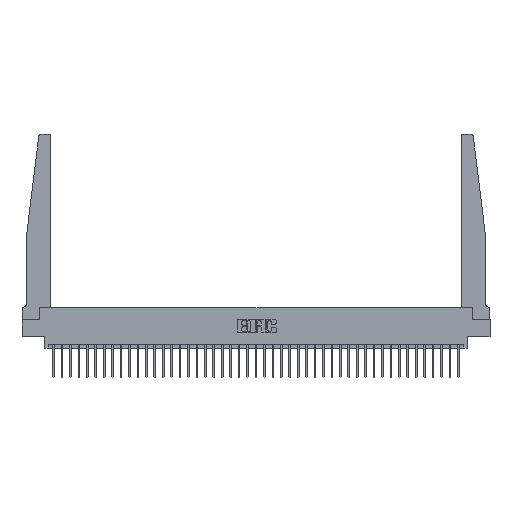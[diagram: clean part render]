
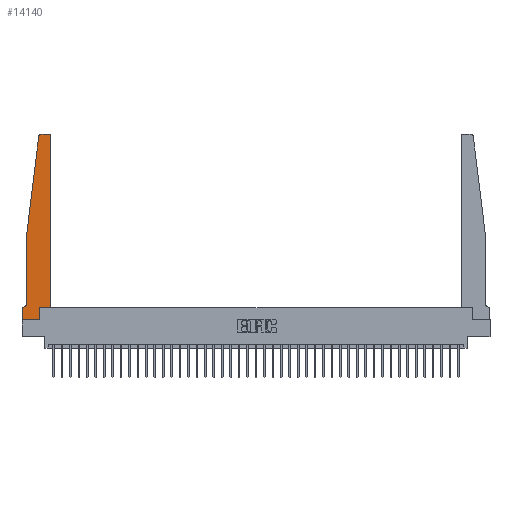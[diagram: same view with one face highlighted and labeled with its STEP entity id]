
A CAD part, top view. The second image highlights one B-rep face of the part: STEP entity #14140.
In plain terms, the highlighted planar face has unit normal (0, 0, 1).
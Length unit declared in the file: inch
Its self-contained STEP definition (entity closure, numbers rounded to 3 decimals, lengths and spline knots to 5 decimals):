
#313 = DIRECTION ( 'NONE',  ( 0., 1., 0. ) ) ;
#480 = EDGE_CURVE ( 'NONE', #21178, #12485, #6880, .T. ) ;
#912 = VERTEX_POINT ( 'NONE', #19153 ) ;
#1433 = DIRECTION ( 'NONE',  ( 0., 0., 1. ) ) ;
#2282 = LINE ( 'NONE', #14441, #31007 ) ;
#2544 = ORIENTED_EDGE ( 'NONE', *, *, #6429, .T. ) ;
#2785 = ORIENTED_EDGE ( 'NONE', *, *, #4045, .T. ) ;
#4045 = EDGE_CURVE ( 'NONE', #18976, #19188, #12335, .T. ) ;
#4588 = ORIENTED_EDGE ( 'NONE', *, *, #19370, .T. ) ;
#4619 = CARTESIAN_POINT ( 'NONE',  ( 0.015, 0.2375, 0.37 ) ) ;
#6387 = LINE ( 'NONE', #34584, #21199 ) ;
#6429 = EDGE_CURVE ( 'NONE', #912, #9850, #34112, .T. ) ;
#6644 = ORIENTED_EDGE ( 'NONE', *, *, #29822, .T. ) ;
#6880 = LINE ( 'NONE', #25906, #16068 ) ;
#7078 = CARTESIAN_POINT ( 'NONE',  ( 0., 0.1875, 0.37 ) ) ;
#7339 = EDGE_CURVE ( 'NONE', #9850, #21178, #26303, .T. ) ;
#7486 = DIRECTION ( 'NONE',  ( -1., 0., 0. ) ) ;
#7758 = CARTESIAN_POINT ( 'NONE',  ( 0.065, 0.2375, 0.37 ) ) ;
#7818 = CARTESIAN_POINT ( 'NONE',  ( 0.2605, 0., 0.37 ) ) ;
#8088 = CARTESIAN_POINT ( 'NONE',  ( 0.065, 1.25, 0.37 ) ) ;
#8310 = FACE_OUTER_BOUND ( 'NONE', #12011, .T. ) ;
#8374 = VECTOR ( 'NONE', #34405, 39.37008 ) ;
#8578 = EDGE_CURVE ( 'NONE', #16094, #34304, #25097, .T. ) ;
#8755 = CARTESIAN_POINT ( 'NONE',  ( 0.425, 0.18, 0.37 ) ) ;
#8774 = AXIS2_PLACEMENT_3D ( 'NONE', #15777, #34956, #18520 ) ;
#9122 = CARTESIAN_POINT ( 'NONE',  ( 0.015, 0.1875, 0.37 ) ) ;
#9349 = DIRECTION ( 'NONE',  ( 1., 0., 0. ) ) ;
#9678 = VERTEX_POINT ( 'NONE', #17785 ) ;
#9850 = VERTEX_POINT ( 'NONE', #7818 ) ;
#10048 = ORIENTED_EDGE ( 'NONE', *, *, #32383, .T. ) ;
#10500 = CARTESIAN_POINT ( 'NONE',  ( 0.065, 0.1875, 0.37 ) ) ;
#11007 = VERTEX_POINT ( 'NONE', #26734 ) ;
#11939 = CARTESIAN_POINT ( 'NONE',  ( 0.2605, 0.18, 0.37 ) ) ;
#12011 = EDGE_LOOP ( 'NONE', ( #32523, #6644, #2785, #13291, #15562, #20922, #10048, #2544, #18389, #19428, #4588, #18630 ) ) ;
#12020 = DIRECTION ( 'NONE',  ( 0., 0., 1. ) ) ;
#12335 = LINE ( 'NONE', #18203, #19683 ) ;
#12485 = VERTEX_POINT ( 'NONE', #8755 ) ;
#13291 = ORIENTED_EDGE ( 'NONE', *, *, #17064, .T. ) ;
#14013 = VECTOR ( 'NONE', #21661, 39.37008 ) ;
#14140 = ADVANCED_FACE ( 'NONE', ( #8310 ), #15522, .T. ) ;
#14441 = CARTESIAN_POINT ( 'NONE',  ( 0.425, 0.18, 0.37 ) ) ;
#14800 = VECTOR ( 'NONE', #31903, 39.37008 ) ;
#15348 = CIRCLE ( 'NONE', #25427, 0.03 ) ;
#15453 = CARTESIAN_POINT ( 'NONE',  ( 0.065, 1.25, 0.37 ) ) ;
#15522 = PLANE ( 'NONE',  #33611 ) ;
#15562 = ORIENTED_EDGE ( 'NONE', *, *, #22036, .T. ) ;
#15777 = CARTESIAN_POINT ( 'NONE',  ( 0.395, 2.72, 0.37 ) ) ;
#15808 = LINE ( 'NONE', #31666, #8374 ) ;
#16068 = VECTOR ( 'NONE', #9349, 39.37008 ) ;
#16094 = VERTEX_POINT ( 'NONE', #29824 ) ;
#16121 = EDGE_CURVE ( 'NONE', #16365, #11007, #29520, .T. ) ;
#16365 = VERTEX_POINT ( 'NONE', #9122 ) ;
#16537 = AXIS2_PLACEMENT_3D ( 'NONE', #4619, #24102, #7486 ) ;
#17064 = EDGE_CURVE ( 'NONE', #19188, #31358, #22991, .T. ) ;
#17785 = CARTESIAN_POINT ( 'NONE',  ( 0.27653, 2.75, 0.37 ) ) ;
#18137 = DIRECTION ( 'NONE',  ( 0., -1., 0. ) ) ;
#18203 = CARTESIAN_POINT ( 'NONE',  ( 0.065, 1.25, 0.37 ) ) ;
#18389 = ORIENTED_EDGE ( 'NONE', *, *, #7339, .T. ) ;
#18520 = DIRECTION ( 'NONE',  ( 1., 0., 0. ) ) ;
#18630 = ORIENTED_EDGE ( 'NONE', *, *, #8578, .T. ) ;
#18976 = VERTEX_POINT ( 'NONE', #34748 ) ;
#19153 = CARTESIAN_POINT ( 'NONE',  ( 0., 0., 0.37 ) ) ;
#19188 = VERTEX_POINT ( 'NONE', #8088 ) ;
#19370 = EDGE_CURVE ( 'NONE', #12485, #16094, #2282, .T. ) ;
#19428 = ORIENTED_EDGE ( 'NONE', *, *, #480, .T. ) ;
#19683 = VECTOR ( 'NONE', #34657, 39.37008 ) ;
#19742 = CARTESIAN_POINT ( 'NONE',  ( 0., 0., 0.37 ) ) ;
#19863 = VECTOR ( 'NONE', #24046, 39.37008 ) ;
#20922 = ORIENTED_EDGE ( 'NONE', *, *, #16121, .T. ) ;
#21063 = DIRECTION ( 'NONE',  ( 1., 0., 0. ) ) ;
#21178 = VERTEX_POINT ( 'NONE', #11939 ) ;
#21199 = VECTOR ( 'NONE', #18137, 39.37008 ) ;
#21276 = CARTESIAN_POINT ( 'NONE',  ( 0.2605, 0.18, 0.37 ) ) ;
#21661 = DIRECTION ( 'NONE',  ( -1., 0., 0. ) ) ;
#22036 = EDGE_CURVE ( 'NONE', #31358, #16365, #23249, .T. ) ;
#22524 = DIRECTION ( 'NONE',  ( 1., 0., 0. ) ) ;
#22991 = LINE ( 'NONE', #15453, #14800 ) ;
#23249 = CIRCLE ( 'NONE', #16537, 0.05 ) ;
#24046 = DIRECTION ( 'NONE',  ( 0., 1., 0. ) ) ;
#24102 = DIRECTION ( 'NONE',  ( 0., 0., -1. ) ) ;
#25097 = CIRCLE ( 'NONE', #8774, 0.03 ) ;
#25427 = AXIS2_PLACEMENT_3D ( 'NONE', #28531, #12020, #31308 ) ;
#25906 = CARTESIAN_POINT ( 'NONE',  ( 0.425, 0.18, 0.37 ) ) ;
#26193 = CARTESIAN_POINT ( 'NONE',  ( 0.395, 2.75, 0.37 ) ) ;
#26303 = LINE ( 'NONE', #21276, #19863 ) ;
#26734 = CARTESIAN_POINT ( 'NONE',  ( 0., 0.1875, 0.37 ) ) ;
#28531 = CARTESIAN_POINT ( 'NONE',  ( 0.27653, 2.72, 0.37 ) ) ;
#29520 = LINE ( 'NONE', #10500, #14013 ) ;
#29631 = EDGE_CURVE ( 'NONE', #34304, #9678, #15808, .T. ) ;
#29822 = EDGE_CURVE ( 'NONE', #9678, #18976, #15348, .T. ) ;
#29824 = CARTESIAN_POINT ( 'NONE',  ( 0.425, 2.72, 0.37 ) ) ;
#31007 = VECTOR ( 'NONE', #313, 39.37008 ) ;
#31308 = DIRECTION ( 'NONE',  ( 1., 0., 0. ) ) ;
#31358 = VERTEX_POINT ( 'NONE', #7758 ) ;
#31666 = CARTESIAN_POINT ( 'NONE',  ( 0.25, 2.75, 0.37 ) ) ;
#31903 = DIRECTION ( 'NONE',  ( 0., -1., 0. ) ) ;
#32383 = EDGE_CURVE ( 'NONE', #11007, #912, #6387, .T. ) ;
#32404 = VECTOR ( 'NONE', #22524, 39.37008 ) ;
#32523 = ORIENTED_EDGE ( 'NONE', *, *, #29631, .T. ) ;
#33611 = AXIS2_PLACEMENT_3D ( 'NONE', #7078, #1433, #21063 ) ;
#34112 = LINE ( 'NONE', #19742, #32404 ) ;
#34304 = VERTEX_POINT ( 'NONE', #26193 ) ;
#34405 = DIRECTION ( 'NONE',  ( -1., 0., 0. ) ) ;
#34584 = CARTESIAN_POINT ( 'NONE',  ( 0., 0., 0.37 ) ) ;
#34657 = DIRECTION ( 'NONE',  ( -0.122, -0.992, 0. ) ) ;
#34748 = CARTESIAN_POINT ( 'NONE',  ( 0.24675, 2.72367, 0.37 ) ) ;
#34956 = DIRECTION ( 'NONE',  ( 0., 0., 1. ) ) ;
